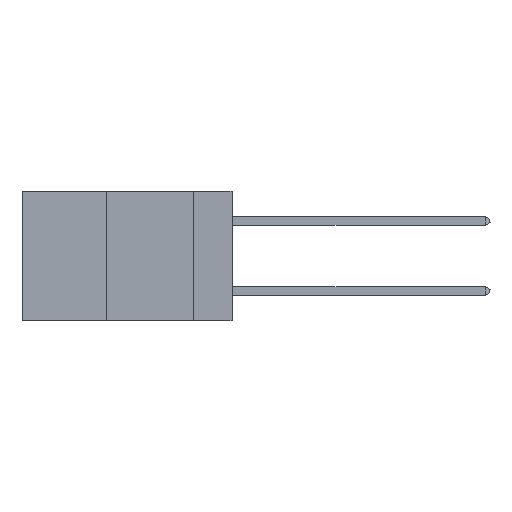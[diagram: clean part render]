
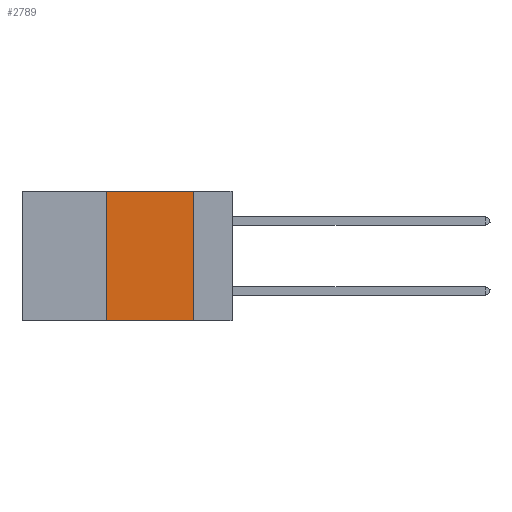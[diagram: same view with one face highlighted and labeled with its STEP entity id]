
A CAD part, left-side view. The second image highlights one B-rep face of the part: STEP entity #2789.
In plain terms, the highlighted planar face has unit normal (-1, 0, 0).
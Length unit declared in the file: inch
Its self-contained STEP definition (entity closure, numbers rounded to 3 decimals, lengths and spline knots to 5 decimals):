
#20 = DIRECTION ( 'NONE',  ( 0., 0., 1. ) ) ;
#23 = ORIENTED_EDGE ( 'NONE', *, *, #594, .F. ) ;
#156 = EDGE_LOOP ( 'NONE', ( #269, #257, #23, #7041 ) ) ;
#257 = ORIENTED_EDGE ( 'NONE', *, *, #3661, .F. ) ;
#269 = ORIENTED_EDGE ( 'NONE', *, *, #11839, .F. ) ;
#594 = EDGE_CURVE ( 'NONE', #1358, #4807, #8200, .T. ) ;
#1116 = DIRECTION ( 'NONE',  ( 0., 0., -1. ) ) ;
#1195 = CARTESIAN_POINT ( 'NONE',  ( 0., 0.11, -0.37 ) ) ;
#1341 = LINE ( 'NONE', #6934, #10975 ) ;
#1358 = VERTEX_POINT ( 'NONE', #4758 ) ;
#1365 = DIRECTION ( 'NONE',  ( 1., 0., 0. ) ) ;
#2140 = DIRECTION ( 'NONE',  ( 0., 0., -1. ) ) ;
#2436 = CARTESIAN_POINT ( 'NONE',  ( 0., 0.11, 0. ) ) ;
#2705 = CARTESIAN_POINT ( 'NONE',  ( 0., 0.6, 0. ) ) ;
#2789 = ADVANCED_FACE ( 'NONE', ( #10577 ), #6827, .F. ) ;
#3079 = CARTESIAN_POINT ( 'NONE',  ( 0., 0.36, 0. ) ) ;
#3661 = EDGE_CURVE ( 'NONE', #4807, #7063, #5763, .T. ) ;
#3825 = VECTOR ( 'NONE', #10583, 39.37008 ) ;
#4093 = CARTESIAN_POINT ( 'NONE',  ( 0., 0.36, 0. ) ) ;
#4758 = CARTESIAN_POINT ( 'NONE',  ( 0., 0.36, -0.37 ) ) ;
#4807 = VERTEX_POINT ( 'NONE', #4093 ) ;
#5127 = DIRECTION ( 'NONE',  ( 0., -1., 0. ) ) ;
#5763 = LINE ( 'NONE', #11133, #3825 ) ;
#6827 = PLANE ( 'NONE',  #7783 ) ;
#6934 = CARTESIAN_POINT ( 'NONE',  ( 0., 0.6, -0.37 ) ) ;
#7041 = ORIENTED_EDGE ( 'NONE', *, *, #8310, .T. ) ;
#7063 = VERTEX_POINT ( 'NONE', #2436 ) ;
#7634 = VERTEX_POINT ( 'NONE', #1195 ) ;
#7783 = AXIS2_PLACEMENT_3D ( 'NONE', #2705, #1365, #2140 ) ;
#8200 = LINE ( 'NONE', #3079, #10012 ) ;
#8299 = VECTOR ( 'NONE', #1116, 39.37008 ) ;
#8310 = EDGE_CURVE ( 'NONE', #1358, #7634, #1341, .T. ) ;
#8722 = CARTESIAN_POINT ( 'NONE',  ( 0., 0.11, 0. ) ) ;
#10012 = VECTOR ( 'NONE', #20, 39.37008 ) ;
#10577 = FACE_OUTER_BOUND ( 'NONE', #156, .T. ) ;
#10583 = DIRECTION ( 'NONE',  ( 0., -1., 0. ) ) ;
#10906 = LINE ( 'NONE', #8722, #8299 ) ;
#10975 = VECTOR ( 'NONE', #5127, 39.37008 ) ;
#11133 = CARTESIAN_POINT ( 'NONE',  ( 0., 0.6, 0. ) ) ;
#11839 = EDGE_CURVE ( 'NONE', #7063, #7634, #10906, .T. ) ;
